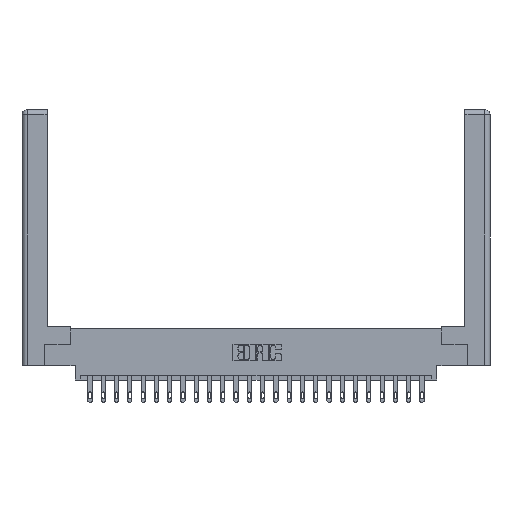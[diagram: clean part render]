
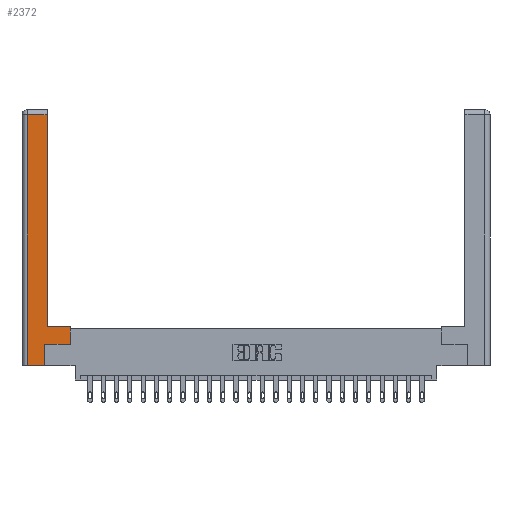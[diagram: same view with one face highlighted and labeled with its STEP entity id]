
A CAD part, top view. The second image highlights one B-rep face of the part: STEP entity #2372.
In plain terms, the highlighted planar face has unit normal (0, 0, 1).
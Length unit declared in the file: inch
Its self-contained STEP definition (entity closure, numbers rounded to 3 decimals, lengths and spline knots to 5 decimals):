
#56 = VERTEX_POINT ( 'NONE', #4441 ) ;
#491 = VECTOR ( 'NONE', #14469, 39.37008 ) ;
#531 = VERTEX_POINT ( 'NONE', #14016 ) ;
#876 = PLANE ( 'NONE',  #7107 ) ;
#1663 = VECTOR ( 'NONE', #9159, 39.37008 ) ;
#1750 = EDGE_CURVE ( 'NONE', #531, #18210, #5012, .T. ) ;
#2372 = ADVANCED_FACE ( 'NONE', ( #8423 ), #876, .F. ) ;
#2465 = VERTEX_POINT ( 'NONE', #5111 ) ;
#2716 = DIRECTION ( 'NONE',  ( 0., 1., 0. ) ) ;
#2934 = CARTESIAN_POINT ( 'NONE',  ( 0.265, 0., 0. ) ) ;
#4172 = EDGE_CURVE ( 'NONE', #18261, #56, #16795, .T. ) ;
#4414 = VECTOR ( 'NONE', #20242, 39.37008 ) ;
#4422 = CARTESIAN_POINT ( 'NONE',  ( 0.295, 0.45, 0. ) ) ;
#4441 = CARTESIAN_POINT ( 'NONE',  ( 0.0615, 2.94, 0. ) ) ;
#4697 = LINE ( 'NONE', #11006, #24521 ) ;
#4868 = EDGE_CURVE ( 'NONE', #10647, #18261, #9830, .T. ) ;
#5012 = LINE ( 'NONE', #16649, #4414 ) ;
#5085 = LINE ( 'NONE', #15109, #13240 ) ;
#5111 = CARTESIAN_POINT ( 'NONE',  ( 0.265, 0.245, 0. ) ) ;
#5343 = LINE ( 'NONE', #8569, #22488 ) ;
#5497 = DIRECTION ( 'NONE',  ( -1., 0., 0. ) ) ;
#5559 = ORIENTED_EDGE ( 'NONE', *, *, #4172, .T. ) ;
#5860 = ORIENTED_EDGE ( 'NONE', *, *, #1750, .T. ) ;
#5901 = ORIENTED_EDGE ( 'NONE', *, *, #14329, .T. ) ;
#6152 = VERTEX_POINT ( 'NONE', #22849 ) ;
#7107 = AXIS2_PLACEMENT_3D ( 'NONE', #14074, #16006, #17913 ) ;
#7188 = DIRECTION ( 'NONE',  ( 0., -1., 0. ) ) ;
#8423 = FACE_OUTER_BOUND ( 'NONE', #22665, .T. ) ;
#8569 = CARTESIAN_POINT ( 'NONE',  ( 0.565, 0.245, 0. ) ) ;
#9159 = DIRECTION ( 'NONE',  ( 0., 1., 0. ) ) ;
#9381 = ORIENTED_EDGE ( 'NONE', *, *, #16251, .T. ) ;
#9574 = CARTESIAN_POINT ( 'NONE',  ( 0.565, 0.45, 0. ) ) ;
#9830 = LINE ( 'NONE', #22528, #1663 ) ;
#10647 = VERTEX_POINT ( 'NONE', #4422 ) ;
#11006 = CARTESIAN_POINT ( 'NONE',  ( 0.0615, 0., 0. ) ) ;
#11303 = ORIENTED_EDGE ( 'NONE', *, *, #21294, .T. ) ;
#12247 = EDGE_CURVE ( 'NONE', #6152, #18328, #13547, .T. ) ;
#12268 = CARTESIAN_POINT ( 'NONE',  ( 0.265, 0.245, 0. ) ) ;
#12453 = DIRECTION ( 'NONE',  ( 1., 0., 0. ) ) ;
#12512 = LINE ( 'NONE', #12268, #16428 ) ;
#13240 = VECTOR ( 'NONE', #5497, 39.37008 ) ;
#13547 = LINE ( 'NONE', #23089, #20134 ) ;
#14016 = CARTESIAN_POINT ( 'NONE',  ( 0.0615, 0., 0. ) ) ;
#14074 = CARTESIAN_POINT ( 'NONE',  ( 0., 0., 0. ) ) ;
#14329 = EDGE_CURVE ( 'NONE', #56, #531, #4697, .T. ) ;
#14395 = EDGE_CURVE ( 'NONE', #18210, #2465, #12512, .T. ) ;
#14469 = DIRECTION ( 'NONE',  ( -1., 0., 0. ) ) ;
#15109 = CARTESIAN_POINT ( 'NONE',  ( 0.295, 0.45, 0. ) ) ;
#16006 = DIRECTION ( 'NONE',  ( 0., 0., -1. ) ) ;
#16251 = EDGE_CURVE ( 'NONE', #2465, #6152, #5343, .T. ) ;
#16384 = ORIENTED_EDGE ( 'NONE', *, *, #12247, .T. ) ;
#16428 = VECTOR ( 'NONE', #2716, 39.37008 ) ;
#16649 = CARTESIAN_POINT ( 'NONE',  ( 0.265, 0., 0. ) ) ;
#16795 = LINE ( 'NONE', #18139, #491 ) ;
#17476 = DIRECTION ( 'NONE',  ( 0., 1., 0. ) ) ;
#17913 = DIRECTION ( 'NONE',  ( -1., 0., 0. ) ) ;
#18139 = CARTESIAN_POINT ( 'NONE',  ( 0.0615, 2.94, 0. ) ) ;
#18210 = VERTEX_POINT ( 'NONE', #2934 ) ;
#18228 = ORIENTED_EDGE ( 'NONE', *, *, #14395, .T. ) ;
#18261 = VERTEX_POINT ( 'NONE', #19248 ) ;
#18328 = VERTEX_POINT ( 'NONE', #9574 ) ;
#19248 = CARTESIAN_POINT ( 'NONE',  ( 0.295, 2.94, 0. ) ) ;
#20134 = VECTOR ( 'NONE', #17476, 39.37008 ) ;
#20242 = DIRECTION ( 'NONE',  ( 1., 0., 0. ) ) ;
#21294 = EDGE_CURVE ( 'NONE', #18328, #10647, #5085, .T. ) ;
#22488 = VECTOR ( 'NONE', #12453, 39.37008 ) ;
#22528 = CARTESIAN_POINT ( 'NONE',  ( 0.295, 3., 0. ) ) ;
#22665 = EDGE_LOOP ( 'NONE', ( #24074, #5559, #5901, #5860, #18228, #9381, #16384, #11303 ) ) ;
#22849 = CARTESIAN_POINT ( 'NONE',  ( 0.565, 0.245, 0. ) ) ;
#23089 = CARTESIAN_POINT ( 'NONE',  ( 0.565, 0.45, 0. ) ) ;
#24074 = ORIENTED_EDGE ( 'NONE', *, *, #4868, .T. ) ;
#24521 = VECTOR ( 'NONE', #7188, 39.37008 ) ;
